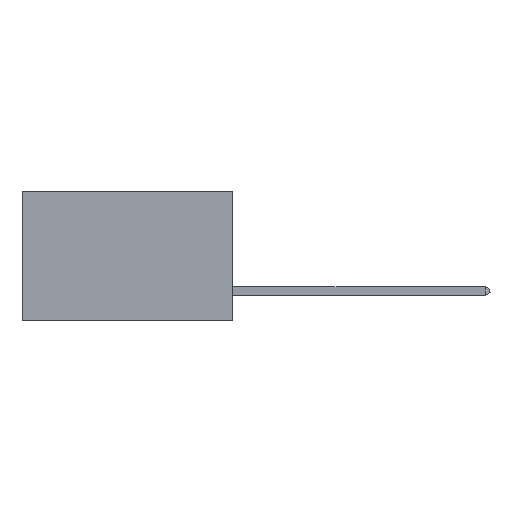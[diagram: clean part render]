
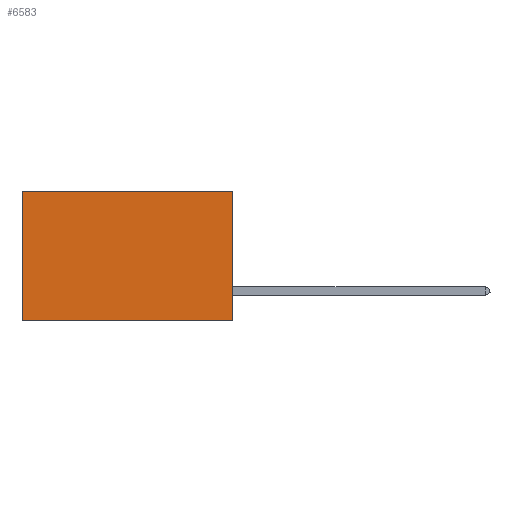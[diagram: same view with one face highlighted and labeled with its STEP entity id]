
A CAD part, left-side view. The second image highlights one B-rep face of the part: STEP entity #6583.
In plain terms, the highlighted planar face has unit normal (-1, 0, 0).
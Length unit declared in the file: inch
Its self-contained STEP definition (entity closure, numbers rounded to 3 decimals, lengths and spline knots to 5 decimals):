
#365 = CARTESIAN_POINT ( 'NONE',  ( 0.2875, 0.6, 0. ) ) ;
#400 = VERTEX_POINT ( 'NONE', #5350 ) ;
#1473 = ORIENTED_EDGE ( 'NONE', *, *, #14602, .T. ) ;
#1717 = VECTOR ( 'NONE', #4173, 39.37008 ) ;
#2423 = EDGE_LOOP ( 'NONE', ( #1473, #13325, #11594, #5476 ) ) ;
#2466 = LINE ( 'NONE', #19297, #1717 ) ;
#3565 = VECTOR ( 'NONE', #8122, 39.37008 ) ;
#3567 = VERTEX_POINT ( 'NONE', #18574 ) ;
#3659 = VECTOR ( 'NONE', #5677, 39.37008 ) ;
#4173 = DIRECTION ( 'NONE',  ( 0., 0., -1. ) ) ;
#5334 = CARTESIAN_POINT ( 'NONE',  ( 0.2875, 0., 0. ) ) ;
#5350 = CARTESIAN_POINT ( 'NONE',  ( 0.2875, 0., 0. ) ) ;
#5476 = ORIENTED_EDGE ( 'NONE', *, *, #12513, .T. ) ;
#5574 = EDGE_CURVE ( 'NONE', #400, #9850, #2466, .T. ) ;
#5677 = DIRECTION ( 'NONE',  ( 0., 1., 0. ) ) ;
#6157 = EDGE_CURVE ( 'NONE', #9850, #14495, #11272, .T. ) ;
#6583 = ADVANCED_FACE ( 'NONE', ( #12226 ), #6832, .F. ) ;
#6832 = PLANE ( 'NONE',  #14710 ) ;
#8122 = DIRECTION ( 'NONE',  ( 0., 0., -1. ) ) ;
#8539 = CARTESIAN_POINT ( 'NONE',  ( 0.2875, 0., -0.37 ) ) ;
#9850 = VERTEX_POINT ( 'NONE', #10246 ) ;
#10021 = DIRECTION ( 'NONE',  ( 1., 0., 0. ) ) ;
#10049 = DIRECTION ( 'NONE',  ( 0., 1., 0. ) ) ;
#10246 = CARTESIAN_POINT ( 'NONE',  ( 0.2875, 0., -0.37 ) ) ;
#11272 = LINE ( 'NONE', #8539, #18273 ) ;
#11594 = ORIENTED_EDGE ( 'NONE', *, *, #5574, .F. ) ;
#11861 = LINE ( 'NONE', #19458, #3659 ) ;
#12226 = FACE_OUTER_BOUND ( 'NONE', #2423, .T. ) ;
#12513 = EDGE_CURVE ( 'NONE', #400, #3567, #11861, .T. ) ;
#13325 = ORIENTED_EDGE ( 'NONE', *, *, #6157, .F. ) ;
#14441 = LINE ( 'NONE', #365, #3565 ) ;
#14495 = VERTEX_POINT ( 'NONE', #14877 ) ;
#14506 = DIRECTION ( 'NONE',  ( 0., 0., -1. ) ) ;
#14602 = EDGE_CURVE ( 'NONE', #3567, #14495, #14441, .T. ) ;
#14710 = AXIS2_PLACEMENT_3D ( 'NONE', #5334, #10021, #14506 ) ;
#14877 = CARTESIAN_POINT ( 'NONE',  ( 0.2875, 0.6, -0.37 ) ) ;
#18273 = VECTOR ( 'NONE', #10049, 39.37008 ) ;
#18574 = CARTESIAN_POINT ( 'NONE',  ( 0.2875, 0.6, 0. ) ) ;
#19297 = CARTESIAN_POINT ( 'NONE',  ( 0.2875, 0., 0. ) ) ;
#19458 = CARTESIAN_POINT ( 'NONE',  ( 0.2875, 0., 0. ) ) ;
